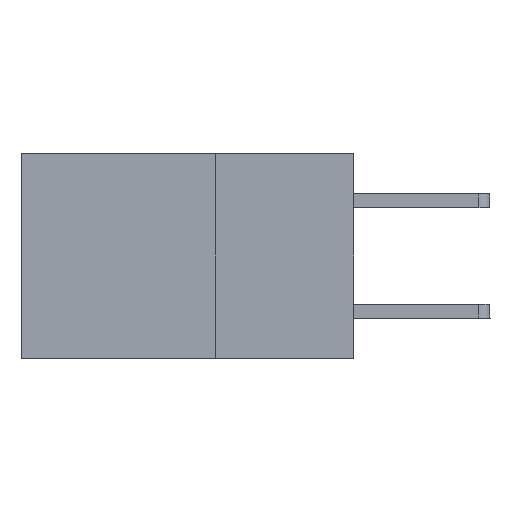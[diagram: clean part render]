
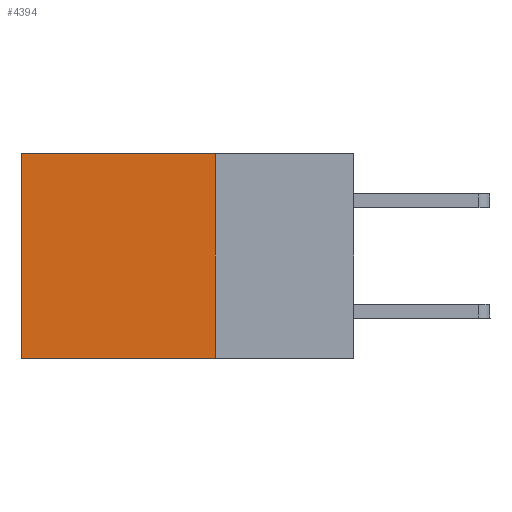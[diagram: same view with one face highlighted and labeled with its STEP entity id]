
A CAD part, left-side view. The second image highlights one B-rep face of the part: STEP entity #4394.
In plain terms, the highlighted planar face has unit normal (-1, 0, 0).
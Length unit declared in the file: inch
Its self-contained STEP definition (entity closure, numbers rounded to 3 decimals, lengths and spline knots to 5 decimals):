
#1641 = LINE ( 'NONE', #3896, #6840 ) ;
#1744 = VERTEX_POINT ( 'NONE', #10451 ) ;
#2126 = EDGE_CURVE ( 'NONE', #6996, #3602, #13729, .T. ) ;
#2422 = VECTOR ( 'NONE', #11863, 39.37008 ) ;
#2766 = DIRECTION ( 'NONE',  ( 0., 0., -1. ) ) ;
#3353 = ORIENTED_EDGE ( 'NONE', *, *, #5735, .T. ) ;
#3602 = VERTEX_POINT ( 'NONE', #8578 ) ;
#3824 = FACE_OUTER_BOUND ( 'NONE', #7465, .T. ) ;
#3896 = CARTESIAN_POINT ( 'NONE',  ( 0.2875, 0.6, 0. ) ) ;
#4095 = EDGE_CURVE ( 'NONE', #1744, #12696, #7574, .T. ) ;
#4201 = ORIENTED_EDGE ( 'NONE', *, *, #6165, .F. ) ;
#4394 = ADVANCED_FACE ( 'NONE', ( #3824 ), #12440, .F. ) ;
#4792 = ORIENTED_EDGE ( 'NONE', *, *, #2126, .T. ) ;
#5591 = AXIS2_PLACEMENT_3D ( 'NONE', #5869, #9114, #2766 ) ;
#5735 = EDGE_CURVE ( 'NONE', #3602, #12696, #1641, .T. ) ;
#5869 = CARTESIAN_POINT ( 'NONE',  ( 0.2875, 0.25, 0. ) ) ;
#6165 = EDGE_CURVE ( 'NONE', #6996, #1744, #12495, .T. ) ;
#6840 = VECTOR ( 'NONE', #8128, 39.37008 ) ;
#6996 = VERTEX_POINT ( 'NONE', #11172 ) ;
#7198 = CARTESIAN_POINT ( 'NONE',  ( 0.2875, 0.25, 0. ) ) ;
#7465 = EDGE_LOOP ( 'NONE', ( #3353, #7974, #4201, #4792 ) ) ;
#7574 = LINE ( 'NONE', #8626, #2422 ) ;
#7974 = ORIENTED_EDGE ( 'NONE', *, *, #4095, .F. ) ;
#8128 = DIRECTION ( 'NONE',  ( 0., 0., -1. ) ) ;
#8146 = CARTESIAN_POINT ( 'NONE',  ( 0.2875, 0.25, 0. ) ) ;
#8578 = CARTESIAN_POINT ( 'NONE',  ( 0.2875, 0.6, 0. ) ) ;
#8626 = CARTESIAN_POINT ( 'NONE',  ( 0.2875, 0.25, -0.37 ) ) ;
#9100 = CARTESIAN_POINT ( 'NONE',  ( 0.2875, 0.6, -0.37 ) ) ;
#9114 = DIRECTION ( 'NONE',  ( 1., 0., 0. ) ) ;
#10451 = CARTESIAN_POINT ( 'NONE',  ( 0.2875, 0.25, -0.37 ) ) ;
#11172 = CARTESIAN_POINT ( 'NONE',  ( 0.2875, 0.25, 0. ) ) ;
#11533 = DIRECTION ( 'NONE',  ( 0., 1., 0. ) ) ;
#11863 = DIRECTION ( 'NONE',  ( 0., 1., 0. ) ) ;
#12352 = DIRECTION ( 'NONE',  ( 0., 0., -1. ) ) ;
#12440 = PLANE ( 'NONE',  #5591 ) ;
#12495 = LINE ( 'NONE', #7198, #13826 ) ;
#12696 = VERTEX_POINT ( 'NONE', #9100 ) ;
#12708 = VECTOR ( 'NONE', #11533, 39.37008 ) ;
#13729 = LINE ( 'NONE', #8146, #12708 ) ;
#13826 = VECTOR ( 'NONE', #12352, 39.37008 ) ;
